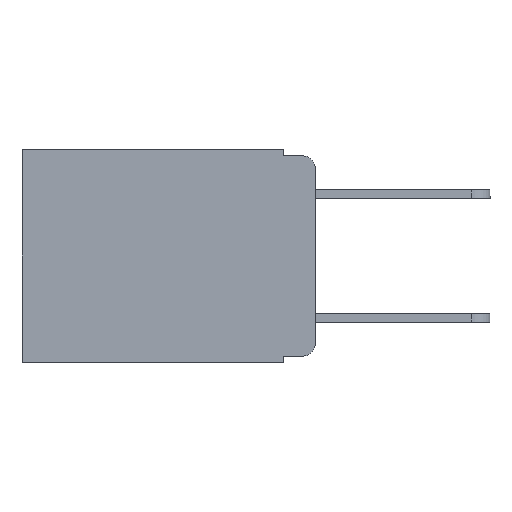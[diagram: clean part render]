
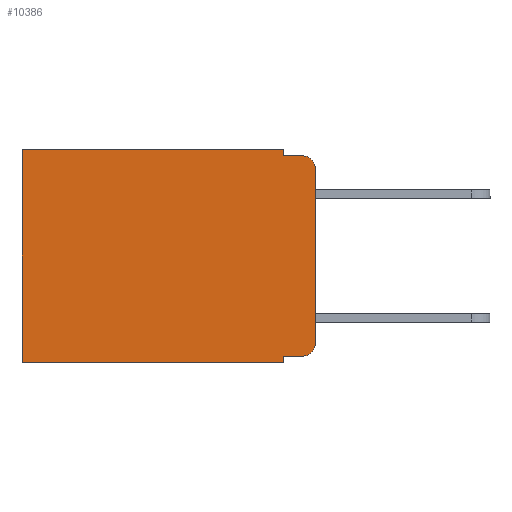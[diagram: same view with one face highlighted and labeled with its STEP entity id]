
A CAD part, left-side view. The second image highlights one B-rep face of the part: STEP entity #10386.
In plain terms, the highlighted planar face has unit normal (-1, 0, 0).
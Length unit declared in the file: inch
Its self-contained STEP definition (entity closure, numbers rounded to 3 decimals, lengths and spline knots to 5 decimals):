
#309 = EDGE_CURVE ( 'NONE', #321, #10164, #5567, .T. ) ;
#321 = VERTEX_POINT ( 'NONE', #9262 ) ;
#470 = EDGE_CURVE ( 'NONE', #4570, #10164, #7538, .T. ) ;
#502 = DIRECTION ( 'NONE',  ( 0., 1., 0. ) ) ;
#556 = VERTEX_POINT ( 'NONE', #8653 ) ;
#640 = VECTOR ( 'NONE', #3271, 39.37008 ) ;
#818 = CARTESIAN_POINT ( 'NONE',  ( 0.298, 0.051, -0.01 ) ) ;
#824 = PLANE ( 'NONE',  #2994 ) ;
#982 = DIRECTION ( 'NONE',  ( 0., -1., 0. ) ) ;
#1157 = EDGE_CURVE ( 'NONE', #556, #4570, #9732, .T. ) ;
#1266 = AXIS2_PLACEMENT_3D ( 'NONE', #9817, #10044, #5447 ) ;
#1459 = DIRECTION ( 'NONE',  ( 0., 0., -1. ) ) ;
#1478 = VECTOR ( 'NONE', #502, 39.37008 ) ;
#1492 = CARTESIAN_POINT ( 'NONE',  ( 0.298, 0., 0. ) ) ;
#1877 = EDGE_LOOP ( 'NONE', ( #9139, #3195, #4640, #5548, #5044, #6480, #5735, #5062, #6990, #4537 ) ) ;
#1942 = LINE ( 'NONE', #4194, #6209 ) ;
#2159 = LINE ( 'NONE', #3666, #6394 ) ;
#2511 = VERTEX_POINT ( 'NONE', #7631 ) ;
#2555 = VERTEX_POINT ( 'NONE', #4634 ) ;
#2685 = DIRECTION ( 'NONE',  ( 0., 0., -1. ) ) ;
#2772 = CARTESIAN_POINT ( 'NONE',  ( 0.298, 0.051, -0.333 ) ) ;
#2881 = CARTESIAN_POINT ( 'NONE',  ( 0.298, 0.02, -0.03 ) ) ;
#2890 = VERTEX_POINT ( 'NONE', #7382 ) ;
#2994 = AXIS2_PLACEMENT_3D ( 'NONE', #3526, #7601, #2685 ) ;
#3195 = ORIENTED_EDGE ( 'NONE', *, *, #309, .T. ) ;
#3271 = DIRECTION ( 'NONE',  ( 0., 1., 0. ) ) ;
#3344 = CARTESIAN_POINT ( 'NONE',  ( 0.298, 0.473, 0. ) ) ;
#3526 = CARTESIAN_POINT ( 'NONE',  ( 0.298, 0., 0. ) ) ;
#3607 = DIRECTION ( 'NONE',  ( -1., 0., 0. ) ) ;
#3666 = CARTESIAN_POINT ( 'NONE',  ( 0.298, 0.051, -0.333 ) ) ;
#3868 = EDGE_CURVE ( 'NONE', #4897, #2890, #2159, .T. ) ;
#3902 = DIRECTION ( 'NONE',  ( 0., 0., -1. ) ) ;
#3924 = DIRECTION ( 'NONE',  ( 0., -1., 0. ) ) ;
#4194 = CARTESIAN_POINT ( 'NONE',  ( 0.298, 0.473, 0. ) ) ;
#4303 = VERTEX_POINT ( 'NONE', #3344 ) ;
#4537 = ORIENTED_EDGE ( 'NONE', *, *, #4555, .T. ) ;
#4555 = EDGE_CURVE ( 'NONE', #2890, #2511, #6396, .T. ) ;
#4570 = VERTEX_POINT ( 'NONE', #818 ) ;
#4634 = CARTESIAN_POINT ( 'NONE',  ( 0.298, 0.473, -0.343 ) ) ;
#4640 = ORIENTED_EDGE ( 'NONE', *, *, #470, .F. ) ;
#4897 = VERTEX_POINT ( 'NONE', #2772 ) ;
#4975 = CARTESIAN_POINT ( 'NONE',  ( 0.298, 0.051, 0. ) ) ;
#5044 = ORIENTED_EDGE ( 'NONE', *, *, #6506, .T. ) ;
#5062 = ORIENTED_EDGE ( 'NONE', *, *, #8557, .F. ) ;
#5355 = DIRECTION ( 'NONE',  ( 0., 0., -1. ) ) ;
#5418 = VECTOR ( 'NONE', #982, 39.37008 ) ;
#5447 = DIRECTION ( 'NONE',  ( 0., 0., -1. ) ) ;
#5548 = ORIENTED_EDGE ( 'NONE', *, *, #1157, .F. ) ;
#5567 = CIRCLE ( 'NONE', #9947, 0.02 ) ;
#5694 = VECTOR ( 'NONE', #3902, 39.37008 ) ;
#5735 = ORIENTED_EDGE ( 'NONE', *, *, #9675, .F. ) ;
#5982 = VECTOR ( 'NONE', #8955, 39.37008 ) ;
#6083 = VECTOR ( 'NONE', #1459, 39.37008 ) ;
#6209 = VECTOR ( 'NONE', #5355, 39.37008 ) ;
#6394 = VECTOR ( 'NONE', #3924, 39.37008 ) ;
#6396 = CIRCLE ( 'NONE', #1266, 0.02 ) ;
#6440 = DIRECTION ( 'NONE',  ( 0., 0., -1. ) ) ;
#6480 = ORIENTED_EDGE ( 'NONE', *, *, #9433, .T. ) ;
#6506 = EDGE_CURVE ( 'NONE', #556, #4303, #7470, .T. ) ;
#6601 = CARTESIAN_POINT ( 'NONE',  ( 0.298, 0., -0.343 ) ) ;
#6895 = VERTEX_POINT ( 'NONE', #10590 ) ;
#6990 = ORIENTED_EDGE ( 'NONE', *, *, #3868, .T. ) ;
#7382 = CARTESIAN_POINT ( 'NONE',  ( 0.298, 0.02, -0.333 ) ) ;
#7427 = CARTESIAN_POINT ( 'NONE',  ( 0.298, 0.051, 0. ) ) ;
#7470 = LINE ( 'NONE', #1492, #640 ) ;
#7538 = LINE ( 'NONE', #8670, #5418 ) ;
#7601 = DIRECTION ( 'NONE',  ( 1., 0., 0. ) ) ;
#7631 = CARTESIAN_POINT ( 'NONE',  ( 0.298, 0., -0.313 ) ) ;
#7855 = LINE ( 'NONE', #6601, #1478 ) ;
#8557 = EDGE_CURVE ( 'NONE', #4897, #6895, #9756, .T. ) ;
#8653 = CARTESIAN_POINT ( 'NONE',  ( 0.298, 0.051, 0. ) ) ;
#8670 = CARTESIAN_POINT ( 'NONE',  ( 0.298, 0.051, -0.01 ) ) ;
#8955 = DIRECTION ( 'NONE',  ( 0., 0., -1. ) ) ;
#9139 = ORIENTED_EDGE ( 'NONE', *, *, #9658, .F. ) ;
#9262 = CARTESIAN_POINT ( 'NONE',  ( 0.298, 0., -0.03 ) ) ;
#9433 = EDGE_CURVE ( 'NONE', #4303, #2555, #1942, .T. ) ;
#9658 = EDGE_CURVE ( 'NONE', #321, #2511, #10297, .T. ) ;
#9675 = EDGE_CURVE ( 'NONE', #6895, #2555, #7855, .T. ) ;
#9732 = LINE ( 'NONE', #7427, #5694 ) ;
#9756 = LINE ( 'NONE', #4975, #5982 ) ;
#9817 = CARTESIAN_POINT ( 'NONE',  ( 0.298, 0.02, -0.313 ) ) ;
#9947 = AXIS2_PLACEMENT_3D ( 'NONE', #2881, #3607, #6440 ) ;
#9961 = FACE_OUTER_BOUND ( 'NONE', #1877, .T. ) ;
#10044 = DIRECTION ( 'NONE',  ( -1., 0., 0. ) ) ;
#10164 = VERTEX_POINT ( 'NONE', #10198 ) ;
#10198 = CARTESIAN_POINT ( 'NONE',  ( 0.298, 0.02, -0.01 ) ) ;
#10297 = LINE ( 'NONE', #10299, #6083 ) ;
#10299 = CARTESIAN_POINT ( 'NONE',  ( 0.298, 0., 0. ) ) ;
#10386 = ADVANCED_FACE ( 'NONE', ( #9961 ), #824, .F. ) ;
#10590 = CARTESIAN_POINT ( 'NONE',  ( 0.298, 0.051, -0.343 ) ) ;
